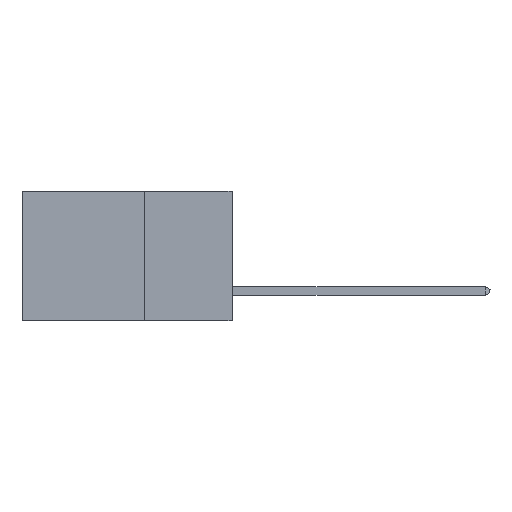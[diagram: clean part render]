
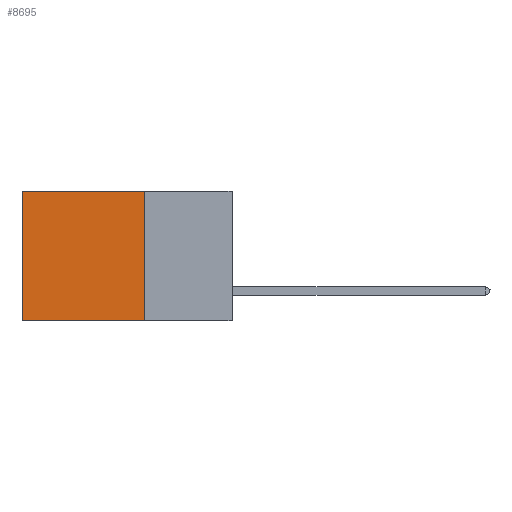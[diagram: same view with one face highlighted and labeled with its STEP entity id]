
A CAD part, left-side view. The second image highlights one B-rep face of the part: STEP entity #8695.
In plain terms, the highlighted planar face has unit normal (-1, 0, 0).
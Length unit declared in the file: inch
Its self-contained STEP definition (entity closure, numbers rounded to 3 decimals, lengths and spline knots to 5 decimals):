
#197 = DIRECTION ( 'NONE',  ( 0., 0., -1. ) ) ;
#735 = VERTEX_POINT ( 'NONE', #35666 ) ;
#1836 = VERTEX_POINT ( 'NONE', #33224 ) ;
#3060 = VECTOR ( 'NONE', #31371, 39.37008 ) ;
#4438 = EDGE_CURVE ( 'NONE', #735, #25396, #18405, .T. ) ;
#4612 = EDGE_LOOP ( 'NONE', ( #35844, #24317, #23923, #6238 ) ) ;
#6238 = ORIENTED_EDGE ( 'NONE', *, *, #13932, .T. ) ;
#8634 = DIRECTION ( 'NONE',  ( 0., 1., 0. ) ) ;
#8695 = ADVANCED_FACE ( 'NONE', ( #12351 ), #25930, .F. ) ;
#11801 = DIRECTION ( 'NONE',  ( 0., 0., -1. ) ) ;
#12351 = FACE_OUTER_BOUND ( 'NONE', #4612, .T. ) ;
#12550 = VECTOR ( 'NONE', #197, 39.37008 ) ;
#13560 = CARTESIAN_POINT ( 'NONE',  ( 0.2875, 0.6, 0. ) ) ;
#13932 = EDGE_CURVE ( 'NONE', #735, #18505, #37715, .T. ) ;
#14237 = VECTOR ( 'NONE', #8634, 39.37008 ) ;
#16612 = CARTESIAN_POINT ( 'NONE',  ( 0.2875, 0.6, 0. ) ) ;
#17595 = CARTESIAN_POINT ( 'NONE',  ( 0.2875, 0.25, -0.37 ) ) ;
#18405 = LINE ( 'NONE', #20952, #27427 ) ;
#18505 = VERTEX_POINT ( 'NONE', #16612 ) ;
#20952 = CARTESIAN_POINT ( 'NONE',  ( 0.2875, 0.25, 0. ) ) ;
#22543 = CARTESIAN_POINT ( 'NONE',  ( 0.2875, 0.25, 0. ) ) ;
#23464 = EDGE_CURVE ( 'NONE', #18505, #1836, #36485, .T. ) ;
#23923 = ORIENTED_EDGE ( 'NONE', *, *, #4438, .F. ) ;
#24317 = ORIENTED_EDGE ( 'NONE', *, *, #28654, .F. ) ;
#25396 = VERTEX_POINT ( 'NONE', #26588 ) ;
#25930 = PLANE ( 'NONE',  #28852 ) ;
#26588 = CARTESIAN_POINT ( 'NONE',  ( 0.2875, 0.25, -0.37 ) ) ;
#27427 = VECTOR ( 'NONE', #11801, 39.37008 ) ;
#28654 = EDGE_CURVE ( 'NONE', #25396, #1836, #37313, .T. ) ;
#28852 = AXIS2_PLACEMENT_3D ( 'NONE', #22543, #35082, #38883 ) ;
#31371 = DIRECTION ( 'NONE',  ( 0., 1., 0. ) ) ;
#33224 = CARTESIAN_POINT ( 'NONE',  ( 0.2875, 0.6, -0.37 ) ) ;
#34734 = CARTESIAN_POINT ( 'NONE',  ( 0.2875, 0.25, 0. ) ) ;
#35082 = DIRECTION ( 'NONE',  ( 1., 0., 0. ) ) ;
#35666 = CARTESIAN_POINT ( 'NONE',  ( 0.2875, 0.25, 0. ) ) ;
#35844 = ORIENTED_EDGE ( 'NONE', *, *, #23464, .T. ) ;
#36485 = LINE ( 'NONE', #13560, #12550 ) ;
#37313 = LINE ( 'NONE', #17595, #3060 ) ;
#37715 = LINE ( 'NONE', #34734, #14237 ) ;
#38883 = DIRECTION ( 'NONE',  ( 0., 0., -1. ) ) ;
